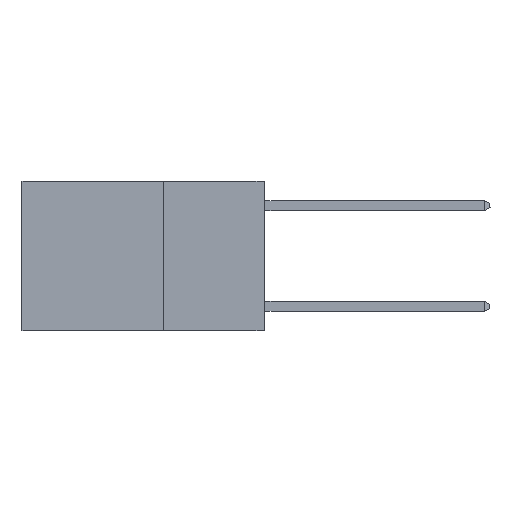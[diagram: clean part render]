
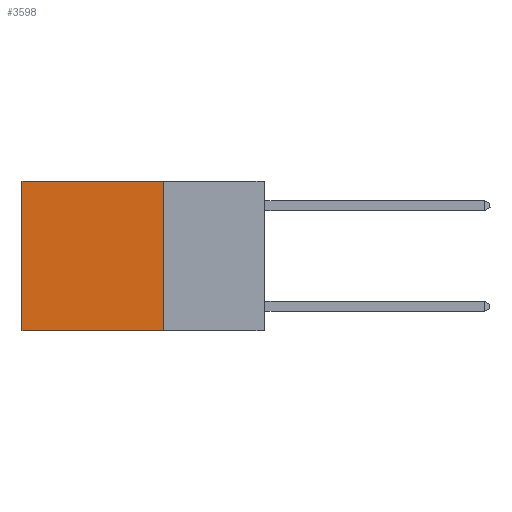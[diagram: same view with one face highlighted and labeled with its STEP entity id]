
A CAD part, left-side view. The second image highlights one B-rep face of the part: STEP entity #3598.
In plain terms, the highlighted planar face has unit normal (-1, 0, 0).
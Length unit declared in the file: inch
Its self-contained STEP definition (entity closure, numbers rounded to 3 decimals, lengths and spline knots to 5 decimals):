
#83 = CARTESIAN_POINT ( 'NONE',  ( 0.2625, 0.25, 0. ) ) ;
#275 = AXIS2_PLACEMENT_3D ( 'NONE', #83, #5487, #14826 ) ;
#1448 = CARTESIAN_POINT ( 'NONE',  ( 0.2625, 0.25, -0.37 ) ) ;
#1522 = CARTESIAN_POINT ( 'NONE',  ( 0.2625, 0.6, -0.37 ) ) ;
#2551 = LINE ( 'NONE', #3812, #12792 ) ;
#2827 = DIRECTION ( 'NONE',  ( 0., 0., -1. ) ) ;
#3598 = ADVANCED_FACE ( 'NONE', ( #11451 ), #16080, .F. ) ;
#3812 = CARTESIAN_POINT ( 'NONE',  ( 0.2625, 0.6, 0. ) ) ;
#3904 = VECTOR ( 'NONE', #8174, 39.37008 ) ;
#4634 = VECTOR ( 'NONE', #16911, 39.37008 ) ;
#4645 = VERTEX_POINT ( 'NONE', #14456 ) ;
#5340 = EDGE_CURVE ( 'NONE', #7726, #5533, #2551, .T. ) ;
#5487 = DIRECTION ( 'NONE',  ( 1., 0., 0. ) ) ;
#5533 = VERTEX_POINT ( 'NONE', #1522 ) ;
#7391 = ORIENTED_EDGE ( 'NONE', *, *, #5340, .T. ) ;
#7726 = VERTEX_POINT ( 'NONE', #14010 ) ;
#7891 = LINE ( 'NONE', #1448, #3904 ) ;
#8113 = EDGE_CURVE ( 'NONE', #4645, #5533, #7891, .T. ) ;
#8174 = DIRECTION ( 'NONE',  ( 0., 1., 0. ) ) ;
#8584 = VECTOR ( 'NONE', #2827, 39.37008 ) ;
#9223 = VERTEX_POINT ( 'NONE', #11734 ) ;
#11451 = FACE_OUTER_BOUND ( 'NONE', #14118, .T. ) ;
#11514 = ORIENTED_EDGE ( 'NONE', *, *, #8113, .F. ) ;
#11734 = CARTESIAN_POINT ( 'NONE',  ( 0.2625, 0.25, 0. ) ) ;
#12792 = VECTOR ( 'NONE', #15802, 39.37008 ) ;
#14010 = CARTESIAN_POINT ( 'NONE',  ( 0.2625, 0.6, 0. ) ) ;
#14118 = EDGE_LOOP ( 'NONE', ( #7391, #11514, #15730, #14140 ) ) ;
#14140 = ORIENTED_EDGE ( 'NONE', *, *, #15965, .T. ) ;
#14456 = CARTESIAN_POINT ( 'NONE',  ( 0.2625, 0.25, -0.37 ) ) ;
#14826 = DIRECTION ( 'NONE',  ( 0., 0., -1. ) ) ;
#14849 = CARTESIAN_POINT ( 'NONE',  ( 0.2625, 0.25, 0. ) ) ;
#15611 = CARTESIAN_POINT ( 'NONE',  ( 0.2625, 0.25, 0. ) ) ;
#15659 = LINE ( 'NONE', #14849, #8584 ) ;
#15693 = LINE ( 'NONE', #15611, #4634 ) ;
#15730 = ORIENTED_EDGE ( 'NONE', *, *, #16868, .F. ) ;
#15802 = DIRECTION ( 'NONE',  ( 0., 0., -1. ) ) ;
#15965 = EDGE_CURVE ( 'NONE', #9223, #7726, #15693, .T. ) ;
#16080 = PLANE ( 'NONE',  #275 ) ;
#16868 = EDGE_CURVE ( 'NONE', #9223, #4645, #15659, .T. ) ;
#16911 = DIRECTION ( 'NONE',  ( 0., 1., 0. ) ) ;
